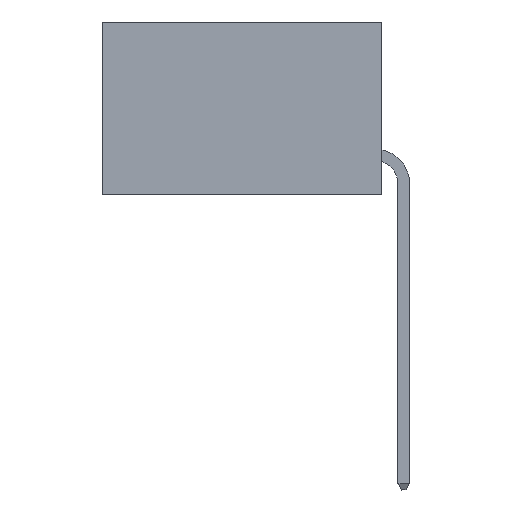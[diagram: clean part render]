
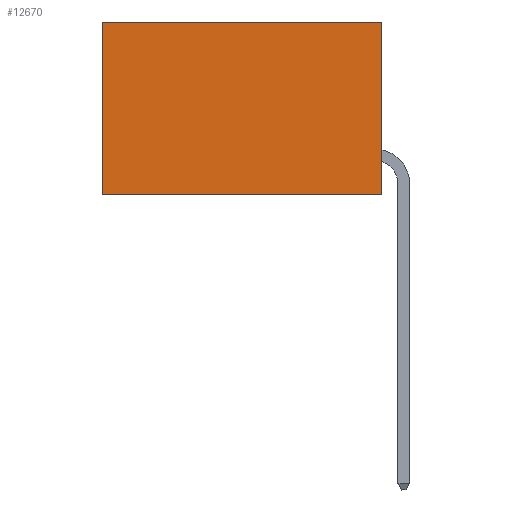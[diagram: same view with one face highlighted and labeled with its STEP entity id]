
A CAD part, left-side view. The second image highlights one B-rep face of the part: STEP entity #12670.
In plain terms, the highlighted planar face has unit normal (-1, 0, 0).
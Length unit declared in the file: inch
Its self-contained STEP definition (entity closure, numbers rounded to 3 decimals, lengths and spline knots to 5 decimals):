
#820 = ORIENTED_EDGE ( 'NONE', *, *, #2390, .T. ) ;
#1537 = VERTEX_POINT ( 'NONE', #9858 ) ;
#1656 = VERTEX_POINT ( 'NONE', #5044 ) ;
#2185 = LINE ( 'NONE', #8111, #5765 ) ;
#2390 = EDGE_CURVE ( 'NONE', #1537, #1656, #2185, .T. ) ;
#3026 = VECTOR ( 'NONE', #8051, 39.37008 ) ;
#3163 = DIRECTION ( 'NONE',  ( 0., 1., 0. ) ) ;
#3452 = FACE_OUTER_BOUND ( 'NONE', #5498, .T. ) ;
#3665 = ORIENTED_EDGE ( 'NONE', *, *, #12781, .T. ) ;
#3988 = ORIENTED_EDGE ( 'NONE', *, *, #10892, .F. ) ;
#4405 = CARTESIAN_POINT ( 'NONE',  ( 0.2875, 0., 0. ) ) ;
#5044 = CARTESIAN_POINT ( 'NONE',  ( 0.2875, 0.6, -0.37 ) ) ;
#5498 = EDGE_LOOP ( 'NONE', ( #820, #9139, #3988, #3665 ) ) ;
#5629 = VERTEX_POINT ( 'NONE', #11656 ) ;
#5765 = VECTOR ( 'NONE', #12251, 39.37008 ) ;
#5812 = CARTESIAN_POINT ( 'NONE',  ( 0.2875, 0., 0. ) ) ;
#6432 = LINE ( 'NONE', #4405, #6589 ) ;
#6589 = VECTOR ( 'NONE', #7496, 39.37008 ) ;
#7471 = VECTOR ( 'NONE', #3163, 39.37008 ) ;
#7496 = DIRECTION ( 'NONE',  ( 0., 0., -1. ) ) ;
#7778 = AXIS2_PLACEMENT_3D ( 'NONE', #5812, #9210, #11206 ) ;
#8051 = DIRECTION ( 'NONE',  ( 0., 1., 0. ) ) ;
#8111 = CARTESIAN_POINT ( 'NONE',  ( 0.2875, 0.6, 0. ) ) ;
#8393 = LINE ( 'NONE', #10939, #7471 ) ;
#8746 = PLANE ( 'NONE',  #7778 ) ;
#9009 = CARTESIAN_POINT ( 'NONE',  ( 0.2875, 0., -0.37 ) ) ;
#9139 = ORIENTED_EDGE ( 'NONE', *, *, #10841, .F. ) ;
#9210 = DIRECTION ( 'NONE',  ( 1., 0., 0. ) ) ;
#9828 = LINE ( 'NONE', #9009, #3026 ) ;
#9858 = CARTESIAN_POINT ( 'NONE',  ( 0.2875, 0.6, 0. ) ) ;
#10623 = CARTESIAN_POINT ( 'NONE',  ( 0.2875, 0., -0.37 ) ) ;
#10841 = EDGE_CURVE ( 'NONE', #11361, #1656, #9828, .T. ) ;
#10892 = EDGE_CURVE ( 'NONE', #5629, #11361, #6432, .T. ) ;
#10939 = CARTESIAN_POINT ( 'NONE',  ( 0.2875, 0., 0. ) ) ;
#11206 = DIRECTION ( 'NONE',  ( 0., 0., -1. ) ) ;
#11361 = VERTEX_POINT ( 'NONE', #10623 ) ;
#11656 = CARTESIAN_POINT ( 'NONE',  ( 0.2875, 0., 0. ) ) ;
#12251 = DIRECTION ( 'NONE',  ( 0., 0., -1. ) ) ;
#12670 = ADVANCED_FACE ( 'NONE', ( #3452 ), #8746, .F. ) ;
#12781 = EDGE_CURVE ( 'NONE', #5629, #1537, #8393, .T. ) ;
